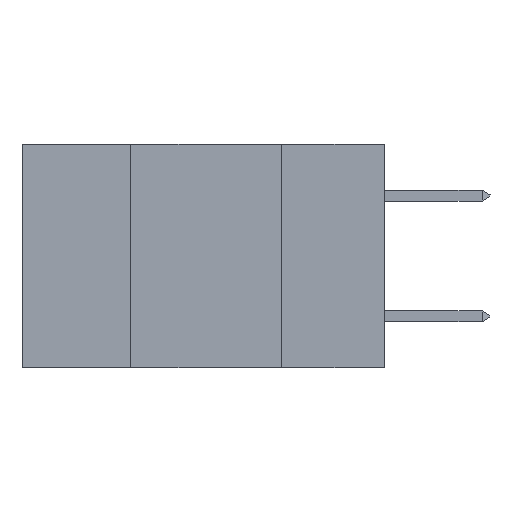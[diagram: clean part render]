
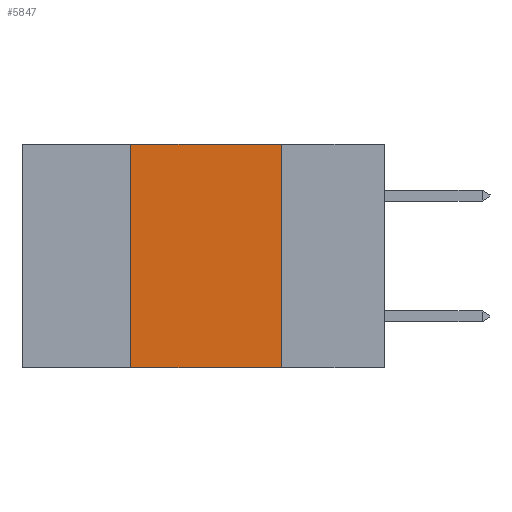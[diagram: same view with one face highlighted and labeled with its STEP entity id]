
A CAD part, left-side view. The second image highlights one B-rep face of the part: STEP entity #5847.
In plain terms, the highlighted planar face has unit normal (-1, 0, 0).
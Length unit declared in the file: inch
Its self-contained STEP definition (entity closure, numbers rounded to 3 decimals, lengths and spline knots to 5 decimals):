
#67 = EDGE_LOOP ( 'NONE', ( #2169, #3976, #10127, #6619 ) ) ;
#490 = VECTOR ( 'NONE', #3628, 39.37008 ) ;
#624 = CARTESIAN_POINT ( 'NONE',  ( 0., 0.6, -0.37 ) ) ;
#666 = FACE_OUTER_BOUND ( 'NONE', #67, .T. ) ;
#830 = CARTESIAN_POINT ( 'NONE',  ( 0., 0.42, 0. ) ) ;
#1118 = AXIS2_PLACEMENT_3D ( 'NONE', #6125, #14451, #7401 ) ;
#1678 = VECTOR ( 'NONE', #1890, 39.37008 ) ;
#1890 = DIRECTION ( 'NONE',  ( 0., -1., 0. ) ) ;
#2169 = ORIENTED_EDGE ( 'NONE', *, *, #14733, .F. ) ;
#2502 = CARTESIAN_POINT ( 'NONE',  ( 0., 0.17, -0.37 ) ) ;
#3137 = CARTESIAN_POINT ( 'NONE',  ( 0., 0.17, 0. ) ) ;
#3486 = DIRECTION ( 'NONE',  ( 0., -1., 0. ) ) ;
#3596 = PLANE ( 'NONE',  #1118 ) ;
#3628 = DIRECTION ( 'NONE',  ( 0., 0., -1. ) ) ;
#3976 = ORIENTED_EDGE ( 'NONE', *, *, #7091, .F. ) ;
#4739 = VECTOR ( 'NONE', #3486, 39.37008 ) ;
#5689 = EDGE_CURVE ( 'NONE', #14925, #5709, #9664, .T. ) ;
#5709 = VERTEX_POINT ( 'NONE', #8398 ) ;
#5847 = ADVANCED_FACE ( 'NONE', ( #666 ), #3596, .F. ) ;
#6125 = CARTESIAN_POINT ( 'NONE',  ( 0., 0.6, 0. ) ) ;
#6249 = VERTEX_POINT ( 'NONE', #3137 ) ;
#6619 = ORIENTED_EDGE ( 'NONE', *, *, #15105, .T. ) ;
#7091 = EDGE_CURVE ( 'NONE', #5709, #6249, #10892, .T. ) ;
#7401 = DIRECTION ( 'NONE',  ( 0., 0., -1. ) ) ;
#8337 = LINE ( 'NONE', #624, #1678 ) ;
#8398 = CARTESIAN_POINT ( 'NONE',  ( 0., 0.42, 0. ) ) ;
#9664 = LINE ( 'NONE', #830, #12395 ) ;
#9858 = CARTESIAN_POINT ( 'NONE',  ( 0., 0.17, 0. ) ) ;
#10127 = ORIENTED_EDGE ( 'NONE', *, *, #5689, .F. ) ;
#10745 = DIRECTION ( 'NONE',  ( 0., 0., 1. ) ) ;
#10892 = LINE ( 'NONE', #10913, #4739 ) ;
#10913 = CARTESIAN_POINT ( 'NONE',  ( 0., 0.6, 0. ) ) ;
#11361 = CARTESIAN_POINT ( 'NONE',  ( 0., 0.42, -0.37 ) ) ;
#12395 = VECTOR ( 'NONE', #10745, 39.37008 ) ;
#12983 = VERTEX_POINT ( 'NONE', #2502 ) ;
#13478 = LINE ( 'NONE', #9858, #490 ) ;
#14451 = DIRECTION ( 'NONE',  ( 1., 0., 0. ) ) ;
#14733 = EDGE_CURVE ( 'NONE', #6249, #12983, #13478, .T. ) ;
#14925 = VERTEX_POINT ( 'NONE', #11361 ) ;
#15105 = EDGE_CURVE ( 'NONE', #14925, #12983, #8337, .T. ) ;
